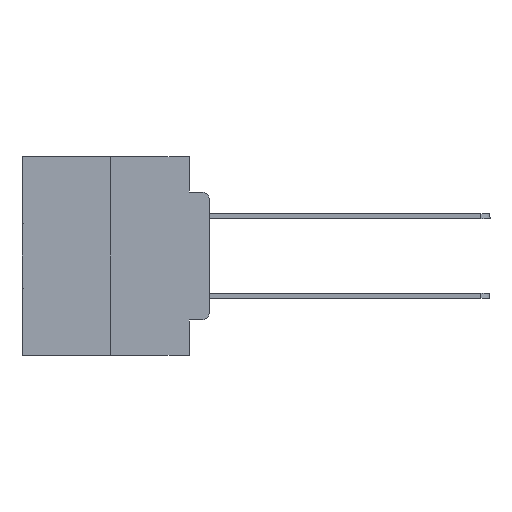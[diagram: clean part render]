
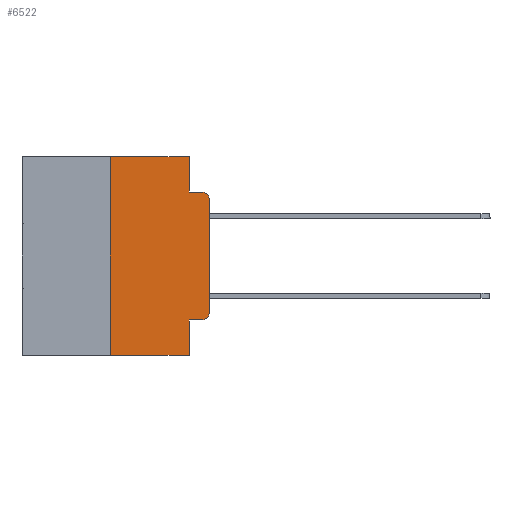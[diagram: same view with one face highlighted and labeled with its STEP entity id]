
A CAD part, left-side view. The second image highlights one B-rep face of the part: STEP entity #6522.
In plain terms, the highlighted planar face has unit normal (-1, 0, 0).
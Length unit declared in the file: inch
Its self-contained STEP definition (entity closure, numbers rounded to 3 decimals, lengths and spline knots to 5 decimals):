
#230 = VECTOR ( 'NONE', #12206, 39.37008 ) ;
#447 = CARTESIAN_POINT ( 'NONE',  ( 0., 0.473, 0. ) ) ;
#3004 = DIRECTION ( 'NONE',  ( 1., 0., 0. ) ) ;
#3122 = EDGE_CURVE ( 'NONE', #10812, #21663, #26024, .T. ) ;
#3358 = VERTEX_POINT ( 'NONE', #5182 ) ;
#4754 = EDGE_CURVE ( 'NONE', #10543, #15403, #13433, .T. ) ;
#5182 = CARTESIAN_POINT ( 'NONE',  ( 0., 0.051, -0.0885 ) ) ;
#5199 = DIRECTION ( 'NONE',  ( -1., 0., 0. ) ) ;
#5273 = VECTOR ( 'NONE', #14127, 39.37008 ) ;
#5427 = VECTOR ( 'NONE', #13761, 39.37008 ) ;
#6103 = CARTESIAN_POINT ( 'NONE',  ( 0., 0., 0. ) ) ;
#6416 = EDGE_CURVE ( 'NONE', #18900, #3358, #10590, .T. ) ;
#6522 = ADVANCED_FACE ( 'NONE', ( #13303 ), #15308, .F. ) ;
#6675 = CARTESIAN_POINT ( 'NONE',  ( 0., 0.473, 0. ) ) ;
#6783 = CARTESIAN_POINT ( 'NONE',  ( 0., 0.25, 0. ) ) ;
#7287 = ORIENTED_EDGE ( 'NONE', *, *, #24701, .T. ) ;
#7424 = CARTESIAN_POINT ( 'NONE',  ( 0., 0.051, 0. ) ) ;
#7979 = VECTOR ( 'NONE', #8589, 39.37008 ) ;
#8589 = DIRECTION ( 'NONE',  ( 0., 0., 1. ) ) ;
#8672 = CARTESIAN_POINT ( 'NONE',  ( 0., 0.02, -0.1085 ) ) ;
#8695 = CARTESIAN_POINT ( 'NONE',  ( 0., 0.473, -0.5 ) ) ;
#8853 = CARTESIAN_POINT ( 'NONE',  ( 0., 0.051, -0.4115 ) ) ;
#9192 = DIRECTION ( 'NONE',  ( 0., 0., -1. ) ) ;
#9616 = CARTESIAN_POINT ( 'NONE',  ( 0., 0., -0.1085 ) ) ;
#9820 = ORIENTED_EDGE ( 'NONE', *, *, #6416, .F. ) ;
#10543 = VERTEX_POINT ( 'NONE', #20025 ) ;
#10590 = LINE ( 'NONE', #7424, #23026 ) ;
#10812 = VERTEX_POINT ( 'NONE', #8853 ) ;
#11148 = DIRECTION ( 'NONE',  ( 0., 0., -1. ) ) ;
#11165 = DIRECTION ( 'NONE',  ( 0., -1., 0. ) ) ;
#11989 = ORIENTED_EDGE ( 'NONE', *, *, #16367, .T. ) ;
#12206 = DIRECTION ( 'NONE',  ( 0., 0., 1. ) ) ;
#12986 = VECTOR ( 'NONE', #16159, 39.37008 ) ;
#13102 = ORIENTED_EDGE ( 'NONE', *, *, #30147, .T. ) ;
#13303 = FACE_OUTER_BOUND ( 'NONE', #14273, .T. ) ;
#13433 = LINE ( 'NONE', #17219, #230 ) ;
#13657 = CARTESIAN_POINT ( 'NONE',  ( 0., 0.051, -0.0885 ) ) ;
#13727 = CARTESIAN_POINT ( 'NONE',  ( 0., 0.051, -0.5 ) ) ;
#13761 = DIRECTION ( 'NONE',  ( 0., -1., 0. ) ) ;
#14127 = DIRECTION ( 'NONE',  ( 0., -1., 0. ) ) ;
#14273 = EDGE_LOOP ( 'NONE', ( #22883, #11989, #19178, #9820, #22126, #23620, #7287, #25073, #13102, #16258 ) ) ;
#14697 = EDGE_CURVE ( 'NONE', #3358, #16619, #25431, .T. ) ;
#14964 = VERTEX_POINT ( 'NONE', #9616 ) ;
#15308 = PLANE ( 'NONE',  #24230 ) ;
#15372 = EDGE_CURVE ( 'NONE', #15403, #18900, #31455, .T. ) ;
#15403 = VERTEX_POINT ( 'NONE', #6783 ) ;
#15647 = CARTESIAN_POINT ( 'NONE',  ( 0., 0.051, 0. ) ) ;
#16159 = DIRECTION ( 'NONE',  ( 0., -1., 0. ) ) ;
#16258 = ORIENTED_EDGE ( 'NONE', *, *, #28526, .T. ) ;
#16367 = EDGE_CURVE ( 'NONE', #14964, #16619, #17618, .T. ) ;
#16575 = CARTESIAN_POINT ( 'NONE',  ( 0., 0.051, 0. ) ) ;
#16577 = VERTEX_POINT ( 'NONE', #21654 ) ;
#16619 = VERTEX_POINT ( 'NONE', #26774 ) ;
#17219 = CARTESIAN_POINT ( 'NONE',  ( 0., 0.25, 0. ) ) ;
#17405 = CIRCLE ( 'NONE', #28303, 0.02 ) ;
#17618 = CIRCLE ( 'NONE', #20920, 0.02 ) ;
#18900 = VERTEX_POINT ( 'NONE', #15647 ) ;
#19178 = ORIENTED_EDGE ( 'NONE', *, *, #14697, .F. ) ;
#19475 = VECTOR ( 'NONE', #9192, 39.37008 ) ;
#19580 = LINE ( 'NONE', #8695, #12986 ) ;
#20025 = CARTESIAN_POINT ( 'NONE',  ( 0., 0.25, -0.5 ) ) ;
#20028 = CARTESIAN_POINT ( 'NONE',  ( 0., 0.02, -0.3915 ) ) ;
#20284 = DIRECTION ( 'NONE',  ( 0., 0., -1. ) ) ;
#20920 = AXIS2_PLACEMENT_3D ( 'NONE', #8672, #25947, #11148 ) ;
#21145 = LINE ( 'NONE', #6103, #7979 ) ;
#21654 = CARTESIAN_POINT ( 'NONE',  ( 0., 0.02, -0.4115 ) ) ;
#21663 = VERTEX_POINT ( 'NONE', #13727 ) ;
#22126 = ORIENTED_EDGE ( 'NONE', *, *, #15372, .F. ) ;
#22251 = DIRECTION ( 'NONE',  ( 0., 0., -1. ) ) ;
#22523 = DIRECTION ( 'NONE',  ( 0., 0., -1. ) ) ;
#22883 = ORIENTED_EDGE ( 'NONE', *, *, #24653, .T. ) ;
#23026 = VECTOR ( 'NONE', #22251, 39.37008 ) ;
#23620 = ORIENTED_EDGE ( 'NONE', *, *, #4754, .F. ) ;
#24230 = AXIS2_PLACEMENT_3D ( 'NONE', #447, #3004, #20284 ) ;
#24653 = EDGE_CURVE ( 'NONE', #25316, #14964, #21145, .T. ) ;
#24701 = EDGE_CURVE ( 'NONE', #10543, #21663, #19580, .T. ) ;
#25073 = ORIENTED_EDGE ( 'NONE', *, *, #3122, .F. ) ;
#25161 = LINE ( 'NONE', #26075, #5427 ) ;
#25316 = VERTEX_POINT ( 'NONE', #25832 ) ;
#25431 = LINE ( 'NONE', #13657, #29603 ) ;
#25832 = CARTESIAN_POINT ( 'NONE',  ( 0., 0., -0.3915 ) ) ;
#25947 = DIRECTION ( 'NONE',  ( -1., 0., 0. ) ) ;
#26024 = LINE ( 'NONE', #16575, #19475 ) ;
#26075 = CARTESIAN_POINT ( 'NONE',  ( 0., 0.051, -0.4115 ) ) ;
#26774 = CARTESIAN_POINT ( 'NONE',  ( 0., 0.02, -0.0885 ) ) ;
#28303 = AXIS2_PLACEMENT_3D ( 'NONE', #20028, #5199, #22523 ) ;
#28526 = EDGE_CURVE ( 'NONE', #16577, #25316, #17405, .T. ) ;
#29603 = VECTOR ( 'NONE', #11165, 39.37008 ) ;
#30147 = EDGE_CURVE ( 'NONE', #10812, #16577, #25161, .T. ) ;
#31455 = LINE ( 'NONE', #6675, #5273 ) ;
